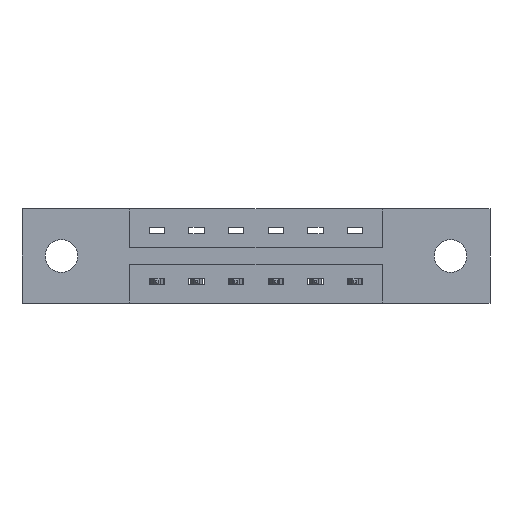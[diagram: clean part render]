
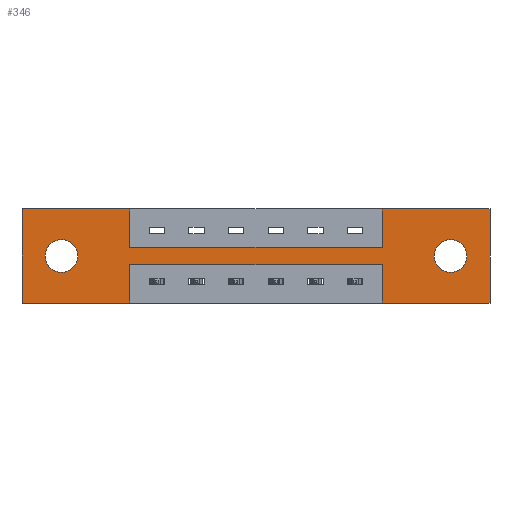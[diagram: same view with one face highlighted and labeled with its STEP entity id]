
A CAD part, front view. The second image highlights one B-rep face of the part: STEP entity #346.
In plain terms, the highlighted planar face has unit normal (0, -1, 0).
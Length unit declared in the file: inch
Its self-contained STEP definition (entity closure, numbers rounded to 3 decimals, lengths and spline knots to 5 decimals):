
#36 = VERTEX_POINT ( 'NONE', #8059 ) ;
#191 = FACE_OUTER_BOUND ( 'NONE', #6707, .T. ) ;
#237 = VECTOR ( 'NONE', #4918, 39.37008 ) ;
#289 = VERTEX_POINT ( 'NONE', #8905 ) ;
#346 = ADVANCED_FACE ( 'NONE', ( #7806, #4503, #191 ), #5434, .T. ) ;
#393 = VERTEX_POINT ( 'NONE', #4883 ) ;
#465 = ORIENTED_EDGE ( 'NONE', *, *, #6779, .F. ) ;
#478 = CARTESIAN_POINT ( 'NONE',  ( 0.425, 0., 0. ) ) ;
#573 = DIRECTION ( 'NONE',  ( 0., 0., 1. ) ) ;
#613 = AXIS2_PLACEMENT_3D ( 'NONE', #7968, #3967, #8538 ) ;
#1085 = ORIENTED_EDGE ( 'NONE', *, *, #6329, .F. ) ;
#1124 = CARTESIAN_POINT ( 'NONE',  ( 0.425, 0., -0.15 ) ) ;
#1146 = VECTOR ( 'NONE', #1529, 39.37008 ) ;
#1232 = DIRECTION ( 'NONE',  ( 1., 0., 0. ) ) ;
#1257 = EDGE_CURVE ( 'NONE', #4469, #7774, #7519, .T. ) ;
#1436 = VERTEX_POINT ( 'NONE', #1721 ) ;
#1529 = DIRECTION ( 'NONE',  ( 0., 0., 1. ) ) ;
#1696 = VERTEX_POINT ( 'NONE', #6787 ) ;
#1713 = VECTOR ( 'NONE', #7626, 39.37008 ) ;
#1721 = CARTESIAN_POINT ( 'NONE',  ( 1.417, 0., -0.22 ) ) ;
#1804 = LINE ( 'NONE', #2359, #7043 ) ;
#1824 = VERTEX_POINT ( 'NONE', #3950 ) ;
#1869 = VECTOR ( 'NONE', #1921, 39.37008 ) ;
#1921 = DIRECTION ( 'NONE',  ( -1., 0., 0. ) ) ;
#1923 = DIRECTION ( 'NONE',  ( 1., 0., 0. ) ) ;
#1957 = LINE ( 'NONE', #6834, #1713 ) ;
#1960 = EDGE_CURVE ( 'NONE', #1696, #36, #2218, .T. ) ;
#2015 = VECTOR ( 'NONE', #1232, 39.37008 ) ;
#2069 = CARTESIAN_POINT ( 'NONE',  ( 0., 0., -0.37 ) ) ;
#2095 = CARTESIAN_POINT ( 'NONE',  ( 0.425, 0., -0.37 ) ) ;
#2218 = CIRCLE ( 'NONE', #5172, 0.064 ) ;
#2264 = VECTOR ( 'NONE', #1923, 39.37008 ) ;
#2275 = DIRECTION ( 'NONE',  ( 0., 0., -1. ) ) ;
#2279 = ORIENTED_EDGE ( 'NONE', *, *, #8062, .T. ) ;
#2293 = VERTEX_POINT ( 'NONE', #6659 ) ;
#2359 = CARTESIAN_POINT ( 'NONE',  ( 0.425, 0., 0. ) ) ;
#2376 = ORIENTED_EDGE ( 'NONE', *, *, #1960, .T. ) ;
#2418 = ORIENTED_EDGE ( 'NONE', *, *, #4542, .F. ) ;
#2449 = ORIENTED_EDGE ( 'NONE', *, *, #3261, .F. ) ;
#2781 = LINE ( 'NONE', #8146, #237 ) ;
#2829 = CARTESIAN_POINT ( 'NONE',  ( 1.687, 0., -0.185 ) ) ;
#2842 = CARTESIAN_POINT ( 'NONE',  ( 1.417, 0., 0. ) ) ;
#2898 = DIRECTION ( 'NONE',  ( 0., 1., 0. ) ) ;
#2994 = CARTESIAN_POINT ( 'NONE',  ( 1.417, 0., -0.15 ) ) ;
#3015 = VERTEX_POINT ( 'NONE', #4690 ) ;
#3149 = CARTESIAN_POINT ( 'NONE',  ( 1.417, 0., -0.37 ) ) ;
#3152 = CARTESIAN_POINT ( 'NONE',  ( 1.842, 0., 0. ) ) ;
#3157 = ORIENTED_EDGE ( 'NONE', *, *, #7197, .F. ) ;
#3188 = EDGE_CURVE ( 'NONE', #7774, #7317, #1957, .T. ) ;
#3211 = EDGE_LOOP ( 'NONE', ( #7017, #2376 ) ) ;
#3261 = EDGE_CURVE ( 'NONE', #7317, #4525, #8248, .T. ) ;
#3262 = LINE ( 'NONE', #3863, #1146 ) ;
#3284 = ORIENTED_EDGE ( 'NONE', *, *, #6097, .T. ) ;
#3558 = ORIENTED_EDGE ( 'NONE', *, *, #5892, .F. ) ;
#3594 = DIRECTION ( 'NONE',  ( 0., -1., 0. ) ) ;
#3635 = CIRCLE ( 'NONE', #7545, 0.064 ) ;
#3765 = VERTEX_POINT ( 'NONE', #3149 ) ;
#3863 = CARTESIAN_POINT ( 'NONE',  ( 1.417, 0., 0. ) ) ;
#3950 = CARTESIAN_POINT ( 'NONE',  ( 0.155, 0., -0.121 ) ) ;
#3967 = DIRECTION ( 'NONE',  ( 0., 1., 0. ) ) ;
#4131 = CARTESIAN_POINT ( 'NONE',  ( 0., 0., -0.37 ) ) ;
#4305 = CARTESIAN_POINT ( 'NONE',  ( 0., 0., 0. ) ) ;
#4469 = VERTEX_POINT ( 'NONE', #2095 ) ;
#4503 = FACE_BOUND ( 'NONE', #6370, .T. ) ;
#4515 = VECTOR ( 'NONE', #8488, 39.37008 ) ;
#4525 = VERTEX_POINT ( 'NONE', #478 ) ;
#4542 = EDGE_CURVE ( 'NONE', #4525, #289, #1804, .T. ) ;
#4690 = CARTESIAN_POINT ( 'NONE',  ( 1.842, 0., 0. ) ) ;
#4856 = LINE ( 'NONE', #4305, #2015 ) ;
#4883 = CARTESIAN_POINT ( 'NONE',  ( 0.155, 0., -0.249 ) ) ;
#4918 = DIRECTION ( 'NONE',  ( 0., 0., 1. ) ) ;
#4976 = DIRECTION ( 'NONE',  ( 1., 0., 0. ) ) ;
#5023 = CARTESIAN_POINT ( 'NONE',  ( 0., 0., 0. ) ) ;
#5172 = AXIS2_PLACEMENT_3D ( 'NONE', #2829, #5357, #8735 ) ;
#5174 = VERTEX_POINT ( 'NONE', #2842 ) ;
#5240 = DIRECTION ( 'NONE',  ( 0., 1., 0. ) ) ;
#5357 = DIRECTION ( 'NONE',  ( 0., 1., 0. ) ) ;
#5388 = LINE ( 'NONE', #7407, #8729 ) ;
#5434 = PLANE ( 'NONE',  #7925 ) ;
#5641 = ORIENTED_EDGE ( 'NONE', *, *, #8298, .F. ) ;
#5709 = DIRECTION ( 'NONE',  ( 0., 0., -1. ) ) ;
#5732 = EDGE_CURVE ( 'NONE', #2293, #3765, #5388, .T. ) ;
#5795 = VECTOR ( 'NONE', #7202, 39.37008 ) ;
#5882 = CIRCLE ( 'NONE', #613, 0.064 ) ;
#5892 = EDGE_CURVE ( 'NONE', #289, #7042, #5895, .T. ) ;
#5895 = LINE ( 'NONE', #1124, #2264 ) ;
#6039 = EDGE_CURVE ( 'NONE', #5174, #3015, #4856, .T. ) ;
#6097 = EDGE_CURVE ( 'NONE', #393, #1824, #3635, .T. ) ;
#6299 = CARTESIAN_POINT ( 'NONE',  ( 0.425, 0., -0.37 ) ) ;
#6329 = EDGE_CURVE ( 'NONE', #7042, #5174, #3262, .T. ) ;
#6370 = EDGE_LOOP ( 'NONE', ( #2279, #3284 ) ) ;
#6464 = ORIENTED_EDGE ( 'NONE', *, *, #1257, .F. ) ;
#6546 = ORIENTED_EDGE ( 'NONE', *, *, #3188, .F. ) ;
#6612 = VECTOR ( 'NONE', #8215, 39.37008 ) ;
#6659 = CARTESIAN_POINT ( 'NONE',  ( 1.842, 0., -0.37 ) ) ;
#6707 = EDGE_LOOP ( 'NONE', ( #8806, #3157, #465, #7038, #5641, #7576, #1085, #3558, #2418, #2449, #6546, #6464 ) ) ;
#6779 = EDGE_CURVE ( 'NONE', #3765, #1436, #2781, .T. ) ;
#6787 = CARTESIAN_POINT ( 'NONE',  ( 1.687, 0., -0.249 ) ) ;
#6834 = CARTESIAN_POINT ( 'NONE',  ( 0., 0., 0. ) ) ;
#7017 = ORIENTED_EDGE ( 'NONE', *, *, #8437, .T. ) ;
#7038 = ORIENTED_EDGE ( 'NONE', *, *, #5732, .F. ) ;
#7042 = VERTEX_POINT ( 'NONE', #2994 ) ;
#7043 = VECTOR ( 'NONE', #2275, 39.37008 ) ;
#7053 = CARTESIAN_POINT ( 'NONE',  ( 0.155, 0., -0.185 ) ) ;
#7197 = EDGE_CURVE ( 'NONE', #1436, #7738, #9044, .T. ) ;
#7202 = DIRECTION ( 'NONE',  ( -1., 0., 0. ) ) ;
#7317 = VERTEX_POINT ( 'NONE', #8001 ) ;
#7407 = CARTESIAN_POINT ( 'NONE',  ( 0., 0., -0.37 ) ) ;
#7519 = LINE ( 'NONE', #4131, #1869 ) ;
#7545 = AXIS2_PLACEMENT_3D ( 'NONE', #7053, #2898, #7709 ) ;
#7576 = ORIENTED_EDGE ( 'NONE', *, *, #6039, .F. ) ;
#7626 = DIRECTION ( 'NONE',  ( 0., 0., 1. ) ) ;
#7644 = EDGE_CURVE ( 'NONE', #7738, #4469, #8285, .T. ) ;
#7666 = CARTESIAN_POINT ( 'NONE',  ( 0.425, 0., -0.22 ) ) ;
#7709 = DIRECTION ( 'NONE',  ( 0., 0., 1. ) ) ;
#7738 = VERTEX_POINT ( 'NONE', #7666 ) ;
#7774 = VERTEX_POINT ( 'NONE', #2069 ) ;
#7806 = FACE_BOUND ( 'NONE', #3211, .T. ) ;
#7821 = LINE ( 'NONE', #3152, #4515 ) ;
#7925 = AXIS2_PLACEMENT_3D ( 'NONE', #8827, #3594, #5709 ) ;
#7968 = CARTESIAN_POINT ( 'NONE',  ( 1.687, 0., -0.185 ) ) ;
#8001 = CARTESIAN_POINT ( 'NONE',  ( 0., 0., 0. ) ) ;
#8059 = CARTESIAN_POINT ( 'NONE',  ( 1.687, 0., -0.121 ) ) ;
#8062 = EDGE_CURVE ( 'NONE', #1824, #393, #8548, .T. ) ;
#8064 = AXIS2_PLACEMENT_3D ( 'NONE', #8940, #5240, #573 ) ;
#8073 = VECTOR ( 'NONE', #4976, 39.37008 ) ;
#8146 = CARTESIAN_POINT ( 'NONE',  ( 1.417, 0., -0.37 ) ) ;
#8215 = DIRECTION ( 'NONE',  ( 0., 0., -1. ) ) ;
#8248 = LINE ( 'NONE', #5023, #8073 ) ;
#8285 = LINE ( 'NONE', #6299, #6612 ) ;
#8298 = EDGE_CURVE ( 'NONE', #3015, #2293, #7821, .T. ) ;
#8437 = EDGE_CURVE ( 'NONE', #36, #1696, #5882, .T. ) ;
#8467 = CARTESIAN_POINT ( 'NONE',  ( 0.425, 0., -0.22 ) ) ;
#8488 = DIRECTION ( 'NONE',  ( 0., 0., -1. ) ) ;
#8538 = DIRECTION ( 'NONE',  ( 0., 0., -1. ) ) ;
#8548 = CIRCLE ( 'NONE', #8064, 0.064 ) ;
#8729 = VECTOR ( 'NONE', #9127, 39.37008 ) ;
#8735 = DIRECTION ( 'NONE',  ( 0., 0., -1. ) ) ;
#8806 = ORIENTED_EDGE ( 'NONE', *, *, #7644, .F. ) ;
#8827 = CARTESIAN_POINT ( 'NONE',  ( 0., 0., -0.37 ) ) ;
#8905 = CARTESIAN_POINT ( 'NONE',  ( 0.425, 0., -0.15 ) ) ;
#8940 = CARTESIAN_POINT ( 'NONE',  ( 0.155, 0., -0.185 ) ) ;
#9044 = LINE ( 'NONE', #8467, #5795 ) ;
#9127 = DIRECTION ( 'NONE',  ( -1., 0., 0. ) ) ;
